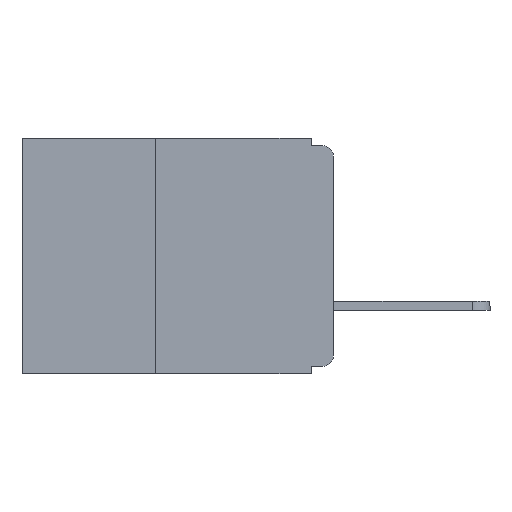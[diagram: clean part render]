
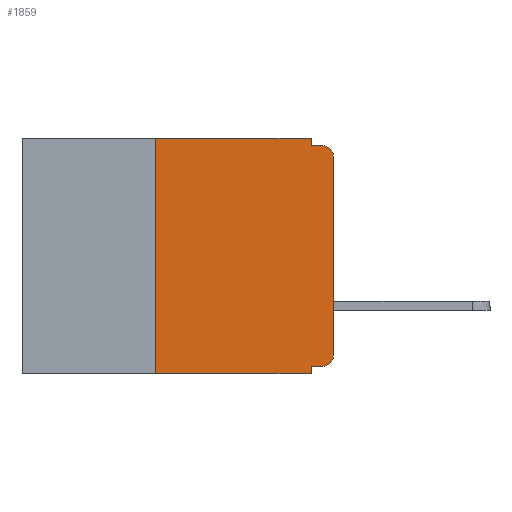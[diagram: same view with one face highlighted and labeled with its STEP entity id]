
A CAD part, left-side view. The second image highlights one B-rep face of the part: STEP entity #1859.
In plain terms, the highlighted planar face has unit normal (-1, 0, 0).
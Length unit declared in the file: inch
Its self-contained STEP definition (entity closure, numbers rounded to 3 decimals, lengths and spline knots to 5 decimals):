
#150 = VECTOR ( 'NONE', #20060, 39.37008 ) ;
#341 = LINE ( 'NONE', #8575, #150 ) ;
#440 = AXIS2_PLACEMENT_3D ( 'NONE', #1926, #1921, #1904 ) ;
#683 = VERTEX_POINT ( 'NONE', #12301 ) ;
#974 = CIRCLE ( 'NONE', #440, 0.015 ) ;
#1417 = VECTOR ( 'NONE', #12958, 39.37008 ) ;
#1439 = LINE ( 'NONE', #12982, #1417 ) ;
#1859 = ADVANCED_FACE ( 'NONE', ( #13730 ), #18758, .F. ) ;
#1904 = DIRECTION ( 'NONE',  ( 0., 0., -1. ) ) ;
#1921 = DIRECTION ( 'NONE',  ( -1., 0., 0. ) ) ;
#1926 = CARTESIAN_POINT ( 'NONE',  ( 0., 0.015, -0.305 ) ) ;
#2253 = ORIENTED_EDGE ( 'NONE', *, *, #7916, .T. ) ;
#2395 = ORIENTED_EDGE ( 'NONE', *, *, #15748, .T. ) ;
#2503 = CARTESIAN_POINT ( 'NONE',  ( 0., 0., 0. ) ) ;
#2673 = ORIENTED_EDGE ( 'NONE', *, *, #15803, .F. ) ;
#2735 = DIRECTION ( 'NONE',  ( 0., -1., 0. ) ) ;
#2875 = ORIENTED_EDGE ( 'NONE', *, *, #4668, .F. ) ;
#2959 = CARTESIAN_POINT ( 'NONE',  ( 0., 0., -0.01 ) ) ;
#3101 = CARTESIAN_POINT ( 'NONE',  ( 0., 0.031, -0.33 ) ) ;
#3112 = CARTESIAN_POINT ( 'NONE',  ( 0., 0.25, 0. ) ) ;
#3180 = ORIENTED_EDGE ( 'NONE', *, *, #4470, .F. ) ;
#3316 = VECTOR ( 'NONE', #9631, 39.37008 ) ;
#3371 = LINE ( 'NONE', #16792, #3316 ) ;
#3420 = ORIENTED_EDGE ( 'NONE', *, *, #6302, .F. ) ;
#3460 = VECTOR ( 'NONE', #2735, 39.37008 ) ;
#3480 = LINE ( 'NONE', #2959, #3460 ) ;
#3498 = VERTEX_POINT ( 'NONE', #16889 ) ;
#3518 = DIRECTION ( 'NONE',  ( 0., 0., 1. ) ) ;
#3624 = VERTEX_POINT ( 'NONE', #3101 ) ;
#3654 = DIRECTION ( 'NONE',  ( 0., 0., -1. ) ) ;
#3658 = DIRECTION ( 'NONE',  ( -1., 0., 0. ) ) ;
#3674 = CARTESIAN_POINT ( 'NONE',  ( 0., 0.015, -0.025 ) ) ;
#3994 = DIRECTION ( 'NONE',  ( 0., 0., -1. ) ) ;
#4069 = ORIENTED_EDGE ( 'NONE', *, *, #12147, .T. ) ;
#4078 = VECTOR ( 'NONE', #14764, 39.37008 ) ;
#4131 = LINE ( 'NONE', #14899, #4078 ) ;
#4182 = ORIENTED_EDGE ( 'NONE', *, *, #16361, .F. ) ;
#4192 = CIRCLE ( 'NONE', #17115, 0.015 ) ;
#4267 = ORIENTED_EDGE ( 'NONE', *, *, #20229, .F. ) ;
#4470 = EDGE_CURVE ( 'NONE', #17434, #18838, #4131, .T. ) ;
#4545 = VERTEX_POINT ( 'NONE', #10126 ) ;
#4643 = ORIENTED_EDGE ( 'NONE', *, *, #13046, .T. ) ;
#4668 = EDGE_CURVE ( 'NONE', #18838, #4545, #3371, .T. ) ;
#5053 = DIRECTION ( 'NONE',  ( 0., -1., 0. ) ) ;
#5326 = VECTOR ( 'NONE', #5053, 39.37008 ) ;
#5340 = LINE ( 'NONE', #5370, #5326 ) ;
#5370 = CARTESIAN_POINT ( 'NONE',  ( 0., 0.437, -0.33 ) ) ;
#6302 = EDGE_CURVE ( 'NONE', #11740, #17434, #341, .T. ) ;
#7436 = AXIS2_PLACEMENT_3D ( 'NONE', #17111, #17325, #3994 ) ;
#7916 = EDGE_CURVE ( 'NONE', #10275, #683, #18421, .T. ) ;
#8459 = CARTESIAN_POINT ( 'NONE',  ( 0., 0.031, -0.33 ) ) ;
#8575 = CARTESIAN_POINT ( 'NONE',  ( 0., 0.25, -0.33 ) ) ;
#8712 = VERTEX_POINT ( 'NONE', #10233 ) ;
#9631 = DIRECTION ( 'NONE',  ( 0., 0., -1. ) ) ;
#10126 = CARTESIAN_POINT ( 'NONE',  ( 0., 0.031, -0.01 ) ) ;
#10233 = CARTESIAN_POINT ( 'NONE',  ( 0., 0.015, -0.01 ) ) ;
#10275 = VERTEX_POINT ( 'NONE', #18895 ) ;
#10333 = DIRECTION ( 'NONE',  ( 0., 0., -1. ) ) ;
#11740 = VERTEX_POINT ( 'NONE', #16910 ) ;
#12147 = EDGE_CURVE ( 'NONE', #11740, #3624, #5340, .T. ) ;
#12301 = CARTESIAN_POINT ( 'NONE',  ( 0., 0., -0.025 ) ) ;
#12958 = DIRECTION ( 'NONE',  ( 0., 1., 0. ) ) ;
#12982 = CARTESIAN_POINT ( 'NONE',  ( 0., 0., -0.32 ) ) ;
#13046 = EDGE_CURVE ( 'NONE', #3498, #10275, #974, .T. ) ;
#13730 = FACE_OUTER_BOUND ( 'NONE', #16631, .T. ) ;
#14764 = DIRECTION ( 'NONE',  ( 0., -1., 0. ) ) ;
#14899 = CARTESIAN_POINT ( 'NONE',  ( 0., 0.437, 0. ) ) ;
#15748 = EDGE_CURVE ( 'NONE', #683, #8712, #4192, .T. ) ;
#15803 = EDGE_CURVE ( 'NONE', #4545, #8712, #3480, .T. ) ;
#16361 = EDGE_CURVE ( 'NONE', #16771, #3624, #16844, .T. ) ;
#16590 = VECTOR ( 'NONE', #10333, 39.37008 ) ;
#16631 = EDGE_LOOP ( 'NONE', ( #2253, #2395, #2673, #2875, #3180, #3420, #4069, #4182, #4267, #4643 ) ) ;
#16771 = VERTEX_POINT ( 'NONE', #16777 ) ;
#16777 = CARTESIAN_POINT ( 'NONE',  ( 0., 0.031, -0.32 ) ) ;
#16792 = CARTESIAN_POINT ( 'NONE',  ( 0., 0.031, 0. ) ) ;
#16844 = LINE ( 'NONE', #8459, #16590 ) ;
#16889 = CARTESIAN_POINT ( 'NONE',  ( 0., 0.015, -0.32 ) ) ;
#16910 = CARTESIAN_POINT ( 'NONE',  ( 0., 0.25, -0.33 ) ) ;
#17111 = CARTESIAN_POINT ( 'NONE',  ( 0., 0.437, 0. ) ) ;
#17115 = AXIS2_PLACEMENT_3D ( 'NONE', #3674, #3658, #3654 ) ;
#17325 = DIRECTION ( 'NONE',  ( 1., 0., 0. ) ) ;
#17434 = VERTEX_POINT ( 'NONE', #3112 ) ;
#18255 = VECTOR ( 'NONE', #3518, 39.37008 ) ;
#18421 = LINE ( 'NONE', #2503, #18255 ) ;
#18758 = PLANE ( 'NONE',  #7436 ) ;
#18838 = VERTEX_POINT ( 'NONE', #19740 ) ;
#18895 = CARTESIAN_POINT ( 'NONE',  ( 0., 0., -0.305 ) ) ;
#19740 = CARTESIAN_POINT ( 'NONE',  ( 0., 0.031, 0. ) ) ;
#20060 = DIRECTION ( 'NONE',  ( 0., 0., 1. ) ) ;
#20229 = EDGE_CURVE ( 'NONE', #3498, #16771, #1439, .T. ) ;
